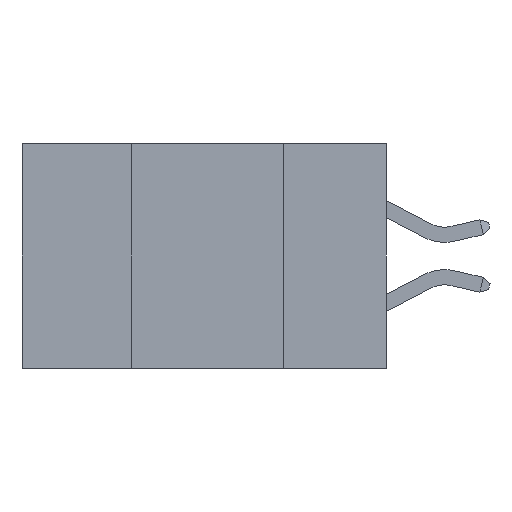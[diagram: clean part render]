
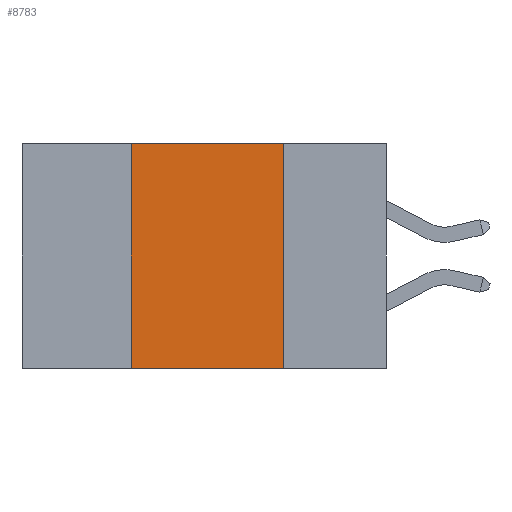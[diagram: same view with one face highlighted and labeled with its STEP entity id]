
A CAD part, left-side view. The second image highlights one B-rep face of the part: STEP entity #8783.
In plain terms, the highlighted planar face has unit normal (-1, 0, 0).
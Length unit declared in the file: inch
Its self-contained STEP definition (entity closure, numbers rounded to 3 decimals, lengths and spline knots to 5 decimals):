
#293 = CARTESIAN_POINT ( 'NONE',  ( 0., 0.42, -0.37 ) ) ;
#419 = EDGE_LOOP ( 'NONE', ( #11480, #644, #4173, #6854 ) ) ;
#644 = ORIENTED_EDGE ( 'NONE', *, *, #9010, .F. ) ;
#1116 = CARTESIAN_POINT ( 'NONE',  ( 0., 0.6, 0. ) ) ;
#1599 = AXIS2_PLACEMENT_3D ( 'NONE', #1116, #17283, #7632 ) ;
#1640 = VERTEX_POINT ( 'NONE', #2104 ) ;
#2104 = CARTESIAN_POINT ( 'NONE',  ( 0., 0.17, 0. ) ) ;
#3707 = LINE ( 'NONE', #16923, #11830 ) ;
#4055 = FACE_OUTER_BOUND ( 'NONE', #419, .T. ) ;
#4173 = ORIENTED_EDGE ( 'NONE', *, *, #4269, .F. ) ;
#4269 = EDGE_CURVE ( 'NONE', #20491, #17450, #3707, .T. ) ;
#4363 = PLANE ( 'NONE',  #1599 ) ;
#4924 = DIRECTION ( 'NONE',  ( 0., -1., 0. ) ) ;
#6553 = DIRECTION ( 'NONE',  ( 0., 0., -1. ) ) ;
#6854 = ORIENTED_EDGE ( 'NONE', *, *, #17674, .T. ) ;
#7632 = DIRECTION ( 'NONE',  ( 0., 0., -1. ) ) ;
#7666 = EDGE_CURVE ( 'NONE', #1640, #20581, #8653, .T. ) ;
#8093 = CARTESIAN_POINT ( 'NONE',  ( 0., 0.17, -0.37 ) ) ;
#8597 = LINE ( 'NONE', #12998, #12410 ) ;
#8653 = LINE ( 'NONE', #8093, #11957 ) ;
#8783 = ADVANCED_FACE ( 'NONE', ( #4055 ), #4363, .F. ) ;
#8885 = DIRECTION ( 'NONE',  ( 0., 0., 1. ) ) ;
#9010 = EDGE_CURVE ( 'NONE', #17450, #1640, #8597, .T. ) ;
#11480 = ORIENTED_EDGE ( 'NONE', *, *, #7666, .F. ) ;
#11728 = CARTESIAN_POINT ( 'NONE',  ( 0., 0.42, 0. ) ) ;
#11830 = VECTOR ( 'NONE', #8885, 39.37008 ) ;
#11844 = CARTESIAN_POINT ( 'NONE',  ( 0., 0.17, -0.37 ) ) ;
#11940 = LINE ( 'NONE', #20267, #19946 ) ;
#11957 = VECTOR ( 'NONE', #6553, 39.37008 ) ;
#12410 = VECTOR ( 'NONE', #4924, 39.37008 ) ;
#12998 = CARTESIAN_POINT ( 'NONE',  ( 0., 0.6, 0. ) ) ;
#16923 = CARTESIAN_POINT ( 'NONE',  ( 0., 0.42, -0.37 ) ) ;
#17283 = DIRECTION ( 'NONE',  ( 1., 0., 0. ) ) ;
#17450 = VERTEX_POINT ( 'NONE', #11728 ) ;
#17674 = EDGE_CURVE ( 'NONE', #20491, #20581, #11940, .T. ) ;
#18680 = DIRECTION ( 'NONE',  ( 0., -1., 0. ) ) ;
#19946 = VECTOR ( 'NONE', #18680, 39.37008 ) ;
#20267 = CARTESIAN_POINT ( 'NONE',  ( 0., 0.6, -0.37 ) ) ;
#20491 = VERTEX_POINT ( 'NONE', #293 ) ;
#20581 = VERTEX_POINT ( 'NONE', #11844 ) ;
